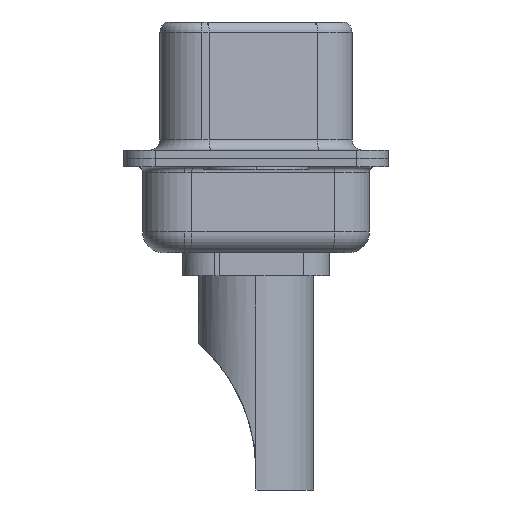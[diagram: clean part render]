
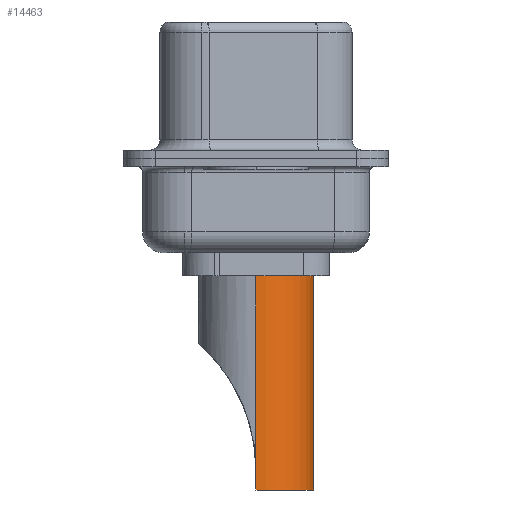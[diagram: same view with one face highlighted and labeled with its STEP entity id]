
A CAD part, left-side view. The second image highlights one B-rep face of the part: STEP entity #14463.
In plain terms, the highlighted cylindrical face has radius 2.75 mm (diameter 5.5 mm), a partial arc.
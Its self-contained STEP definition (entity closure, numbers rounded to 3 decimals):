
#354 = CIRCLE ( 'NONE', #1940, 2.75 ) ;
#522 = DIRECTION ( 'NONE',  ( 0., 0., 1. ) ) ;
#1098 = CARTESIAN_POINT ( 'NONE',  ( 0., 0., 4.234 ) ) ;
#1279 = CARTESIAN_POINT ( 'NONE',  ( 2.75, 0., -8.7 ) ) ;
#1464 = ORIENTED_EDGE ( 'NONE', *, *, #15512, .T. ) ;
#1940 = AXIS2_PLACEMENT_3D ( 'NONE', #11271, #522, #10014 ) ;
#2619 = CARTESIAN_POINT ( 'NONE',  ( 2.75, 0., 1.5 ) ) ;
#2628 = DIRECTION ( 'NONE',  ( 0., 0., 1. ) ) ;
#3481 = LINE ( 'NONE', #16125, #13017 ) ;
#3495 = CARTESIAN_POINT ( 'NONE',  ( -2.75, 0., -7.764 ) ) ;
#3731 = DIRECTION ( 'NONE',  ( 0., 0., 1. ) ) ;
#4235 = ORIENTED_EDGE ( 'NONE', *, *, #14261, .F. ) ;
#4679 = ORIENTED_EDGE ( 'NONE', *, *, #14038, .F. ) ;
#5254 = VECTOR ( 'NONE', #3731, 1000. ) ;
#5824 = DIRECTION ( 'NONE',  ( 0., 0., 1. ) ) ;
#6040 = CARTESIAN_POINT ( 'NONE',  ( 2.75, 0., -7.764 ) ) ;
#6305 = LINE ( 'NONE', #1279, #8812 ) ;
#6317 = VERTEX_POINT ( 'NONE', #9343 ) ;
#6571 = ORIENTED_EDGE ( 'NONE', *, *, #15397, .T. ) ;
#6696 = LINE ( 'NONE', #10137, #13692 ) ;
#6839 = DIRECTION ( 'NONE',  ( 0., 0., -1. ) ) ;
#6972 = AXIS2_PLACEMENT_3D ( 'NONE', #12498, #5824, #6985 ) ;
#6985 = DIRECTION ( 'NONE',  ( 1., 0., 0. ) ) ;
#7190 = ORIENTED_EDGE ( 'NONE', *, *, #14812, .F. ) ;
#7371 = CARTESIAN_POINT ( 'NONE',  ( -2.75, 0., 1.5 ) ) ;
#7402 = VERTEX_POINT ( 'NONE', #7371 ) ;
#7910 = CARTESIAN_POINT ( 'NONE',  ( -2.75, 0., 4.234 ) ) ;
#7973 = CYLINDRICAL_SURFACE ( 'NONE', #10499, 2.75 ) ;
#8076 = DIRECTION ( 'NONE',  ( 1., 0., 0. ) ) ;
#8176 = DIRECTION ( 'NONE',  ( 0., 0., 1. ) ) ;
#8812 = VECTOR ( 'NONE', #6839, 1000. ) ;
#9343 = CARTESIAN_POINT ( 'NONE',  ( 2.75, 0., -8.7 ) ) ;
#10014 = DIRECTION ( 'NONE',  ( 1., 0., 0. ) ) ;
#10137 = CARTESIAN_POINT ( 'NONE',  ( -2.75, 0., -8.7 ) ) ;
#10148 = LINE ( 'NONE', #7910, #5254 ) ;
#10499 = AXIS2_PLACEMENT_3D ( 'NONE', #1098, #2628, #8076 ) ;
#11271 = CARTESIAN_POINT ( 'NONE',  ( 0., 0., 1.5 ) ) ;
#11365 = CIRCLE ( 'NONE', #6972, 2.75 ) ;
#11431 = ORIENTED_EDGE ( 'NONE', *, *, #16878, .T. ) ;
#12261 = VERTEX_POINT ( 'NONE', #2619 ) ;
#12488 = VERTEX_POINT ( 'NONE', #6040 ) ;
#12498 = CARTESIAN_POINT ( 'NONE',  ( 0., 0., -8.7 ) ) ;
#13017 = VECTOR ( 'NONE', #8176, 1000. ) ;
#13692 = VECTOR ( 'NONE', #15692, 1000. ) ;
#14038 = EDGE_CURVE ( 'NONE', #7402, #12261, #354, .T. ) ;
#14261 = EDGE_CURVE ( 'NONE', #17203, #7402, #10148, .T. ) ;
#14463 = ADVANCED_FACE ( 'NONE', ( #15894 ), #7973, .T. ) ;
#14545 = VERTEX_POINT ( 'NONE', #16390 ) ;
#14812 = EDGE_CURVE ( 'NONE', #12488, #6317, #6305, .T. ) ;
#15397 = EDGE_CURVE ( 'NONE', #14545, #6317, #11365, .T. ) ;
#15512 = EDGE_CURVE ( 'NONE', #17203, #14545, #6696, .T. ) ;
#15692 = DIRECTION ( 'NONE',  ( 0., 0., -1. ) ) ;
#15751 = EDGE_LOOP ( 'NONE', ( #4235, #1464, #6571, #7190, #11431, #4679 ) ) ;
#15894 = FACE_OUTER_BOUND ( 'NONE', #15751, .T. ) ;
#16125 = CARTESIAN_POINT ( 'NONE',  ( 2.75, 0., 4.234 ) ) ;
#16390 = CARTESIAN_POINT ( 'NONE',  ( -2.75, 0., -8.7 ) ) ;
#16878 = EDGE_CURVE ( 'NONE', #12488, #12261, #3481, .T. ) ;
#17203 = VERTEX_POINT ( 'NONE', #3495 ) ;
